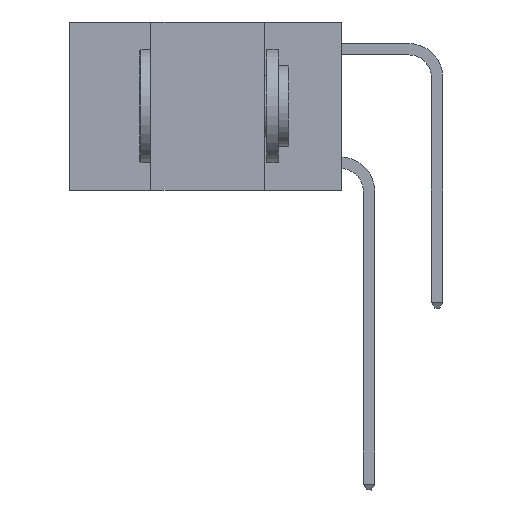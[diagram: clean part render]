
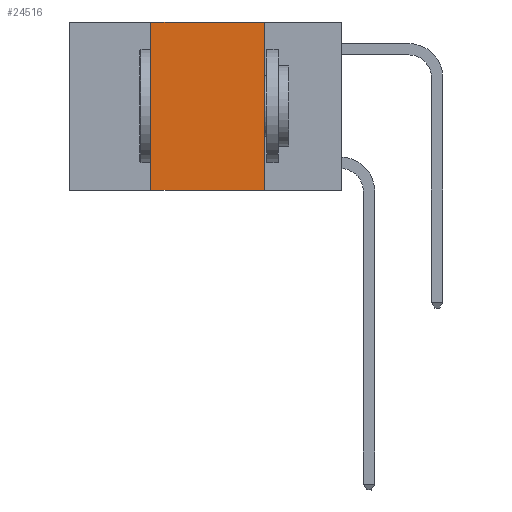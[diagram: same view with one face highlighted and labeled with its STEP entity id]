
A CAD part, left-side view. The second image highlights one B-rep face of the part: STEP entity #24516.
In plain terms, the highlighted planar face has unit normal (-1, 0, 0).
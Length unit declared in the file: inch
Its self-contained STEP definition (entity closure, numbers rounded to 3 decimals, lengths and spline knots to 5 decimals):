
#837 = ORIENTED_EDGE ( 'NONE', *, *, #26475, .T. ) ;
#1087 = LINE ( 'NONE', #10596, #12599 ) ;
#1782 = CARTESIAN_POINT ( 'NONE',  ( 0., 0.17, -0.37 ) ) ;
#4056 = DIRECTION ( 'NONE',  ( 1., 0., 0. ) ) ;
#6770 = EDGE_LOOP ( 'NONE', ( #17618, #17699, #24452, #837 ) ) ;
#7407 = CARTESIAN_POINT ( 'NONE',  ( 0., 0.17, 0. ) ) ;
#7842 = AXIS2_PLACEMENT_3D ( 'NONE', #11032, #4056, #28790 ) ;
#8599 = VERTEX_POINT ( 'NONE', #1782 ) ;
#9483 = DIRECTION ( 'NONE',  ( 0., -1., 0. ) ) ;
#9780 = CARTESIAN_POINT ( 'NONE',  ( 0., 0.6, 0. ) ) ;
#10596 = CARTESIAN_POINT ( 'NONE',  ( 0., 0.17, 0. ) ) ;
#10857 = DIRECTION ( 'NONE',  ( 0., 0., -1. ) ) ;
#10880 = FACE_OUTER_BOUND ( 'NONE', #6770, .T. ) ;
#11032 = CARTESIAN_POINT ( 'NONE',  ( 0., 0.6, 0. ) ) ;
#11687 = DIRECTION ( 'NONE',  ( 0., 0., 1. ) ) ;
#11896 = CARTESIAN_POINT ( 'NONE',  ( 0., 0.42, 0. ) ) ;
#12599 = VECTOR ( 'NONE', #10857, 39.37008 ) ;
#12851 = CARTESIAN_POINT ( 'NONE',  ( 0., 0.6, -0.37 ) ) ;
#13033 = VECTOR ( 'NONE', #15050, 39.37008 ) ;
#14402 = EDGE_CURVE ( 'NONE', #24886, #17626, #25187, .T. ) ;
#15050 = DIRECTION ( 'NONE',  ( 0., -1., 0. ) ) ;
#15202 = EDGE_CURVE ( 'NONE', #17710, #24886, #25130, .T. ) ;
#15733 = VECTOR ( 'NONE', #11687, 39.37008 ) ;
#17548 = PLANE ( 'NONE',  #7842 ) ;
#17618 = ORIENTED_EDGE ( 'NONE', *, *, #25483, .F. ) ;
#17626 = VERTEX_POINT ( 'NONE', #7407 ) ;
#17699 = ORIENTED_EDGE ( 'NONE', *, *, #14402, .F. ) ;
#17710 = VERTEX_POINT ( 'NONE', #25422 ) ;
#21408 = CARTESIAN_POINT ( 'NONE',  ( 0., 0.42, 0. ) ) ;
#23804 = VECTOR ( 'NONE', #9483, 39.37008 ) ;
#24452 = ORIENTED_EDGE ( 'NONE', *, *, #15202, .F. ) ;
#24516 = ADVANCED_FACE ( 'NONE', ( #10880 ), #17548, .F. ) ;
#24886 = VERTEX_POINT ( 'NONE', #21408 ) ;
#25130 = LINE ( 'NONE', #11896, #15733 ) ;
#25187 = LINE ( 'NONE', #9780, #23804 ) ;
#25294 = LINE ( 'NONE', #12851, #13033 ) ;
#25422 = CARTESIAN_POINT ( 'NONE',  ( 0., 0.42, -0.37 ) ) ;
#25483 = EDGE_CURVE ( 'NONE', #17626, #8599, #1087, .T. ) ;
#26475 = EDGE_CURVE ( 'NONE', #17710, #8599, #25294, .T. ) ;
#28790 = DIRECTION ( 'NONE',  ( 0., 0., -1. ) ) ;
